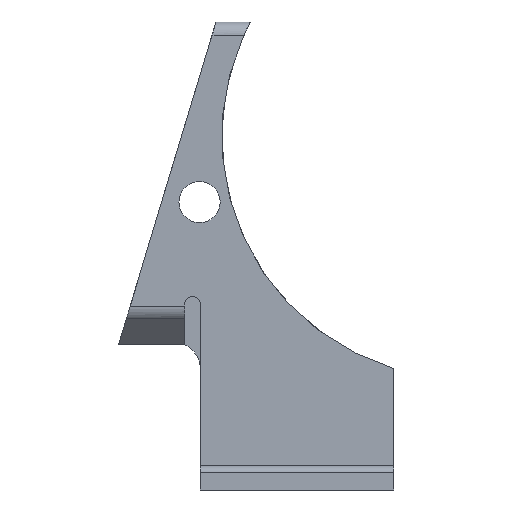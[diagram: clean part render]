
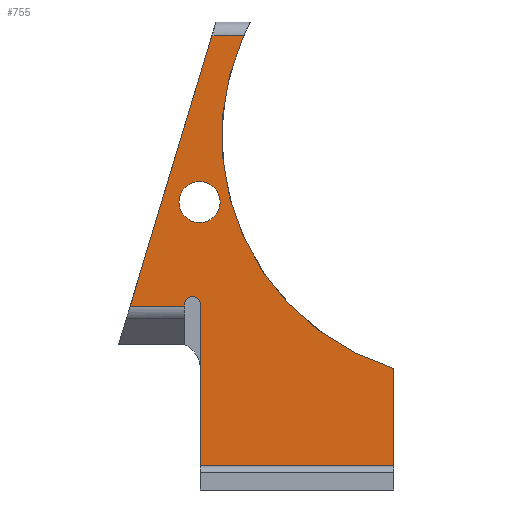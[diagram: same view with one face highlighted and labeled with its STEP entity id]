
A CAD part, left-side view. The second image highlights one B-rep face of the part: STEP entity #755.
In plain terms, the highlighted planar face has unit normal (-1, 0, 0).
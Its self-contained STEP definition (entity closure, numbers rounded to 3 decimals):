
#19=FACE_BOUND('',#89,.T.);
#24=PLANE('',#816);
#48=FACE_OUTER_BOUND('',#88,.T.);
#88=EDGE_LOOP('',(#528,#529,#530,#531,#532,#533,#534,#535,#536,#537,#538));
#89=EDGE_LOOP('',(#539));
#131=CIRCLE('',#817,0.5);
#132=CIRCLE('',#818,0.5);
#133=CIRCLE('',#819,17.951);
#134=CIRCLE('',#820,1.525);
#157=LINE('',#1112,#235);
#158=LINE('',#1115,#236);
#168=LINE('',#1145,#246);
#169=LINE('',#1149,#247);
#170=LINE('',#1153,#248);
#171=LINE('',#1155,#249);
#172=LINE('',#1157,#250);
#173=LINE('',#1160,#251);
#235=VECTOR('',#888,10.);
#236=VECTOR('',#891,10.);
#246=VECTOR('',#913,10.);
#247=VECTOR('',#916,10.);
#248=VECTOR('',#919,10.);
#249=VECTOR('',#920,10.);
#250=VECTOR('',#921,10.);
#251=VECTOR('',#924,10.);
#318=VERTEX_POINT('',#1105);
#321=VERTEX_POINT('',#1110);
#322=VERTEX_POINT('',#1114);
#336=VERTEX_POINT('',#1144);
#337=VERTEX_POINT('',#1146);
#338=VERTEX_POINT('',#1148);
#339=VERTEX_POINT('',#1150);
#340=VERTEX_POINT('',#1152);
#341=VERTEX_POINT('',#1154);
#342=VERTEX_POINT('',#1156);
#343=VERTEX_POINT('',#1158);
#344=VERTEX_POINT('',#1161);
#397=EDGE_CURVE('',#321,#318,#157,.T.);
#398=EDGE_CURVE('',#322,#318,#158,.T.);
#413=EDGE_CURVE('',#321,#336,#168,.T.);
#414=EDGE_CURVE('',#336,#337,#131,.T.);
#415=EDGE_CURVE('',#337,#338,#169,.T.);
#416=EDGE_CURVE('',#338,#339,#132,.T.);
#417=EDGE_CURVE('',#339,#340,#170,.T.);
#418=EDGE_CURVE('',#341,#340,#171,.T.);
#419=EDGE_CURVE('',#342,#341,#172,.T.);
#420=EDGE_CURVE('',#342,#343,#133,.T.);
#421=EDGE_CURVE('',#322,#343,#173,.T.);
#422=EDGE_CURVE('',#344,#344,#134,.T.);
#528=ORIENTED_EDGE('',*,*,#397,.F.);
#529=ORIENTED_EDGE('',*,*,#413,.T.);
#530=ORIENTED_EDGE('',*,*,#414,.T.);
#531=ORIENTED_EDGE('',*,*,#415,.T.);
#532=ORIENTED_EDGE('',*,*,#416,.T.);
#533=ORIENTED_EDGE('',*,*,#417,.T.);
#534=ORIENTED_EDGE('',*,*,#418,.F.);
#535=ORIENTED_EDGE('',*,*,#419,.F.);
#536=ORIENTED_EDGE('',*,*,#420,.T.);
#537=ORIENTED_EDGE('',*,*,#421,.F.);
#538=ORIENTED_EDGE('',*,*,#398,.T.);
#539=ORIENTED_EDGE('',*,*,#422,.T.);
#755=ADVANCED_FACE('',(#48,#19),#24,.T.);
#816=AXIS2_PLACEMENT_3D('',#1143,#911,#912);
#817=AXIS2_PLACEMENT_3D('',#1147,#914,#915);
#818=AXIS2_PLACEMENT_3D('',#1151,#917,#918);
#819=AXIS2_PLACEMENT_3D('',#1159,#922,#923);
#820=AXIS2_PLACEMENT_3D('',#1162,#925,#926);
#888=DIRECTION('',(0.,1.,0.));
#891=DIRECTION('',(0.,0.289,-0.957));
#911=DIRECTION('center_axis',(-1.,0.,0.));
#912=DIRECTION('ref_axis',(0.,0.,1.));
#913=DIRECTION('',(0.,0.,1.));
#914=DIRECTION('center_axis',(1.,0.,0.));
#915=DIRECTION('ref_axis',(0.,-1.,0.));
#916=DIRECTION('',(0.,-1.,0.));
#917=DIRECTION('center_axis',(1.,0.,0.));
#918=DIRECTION('ref_axis',(0.,-1.,0.));
#919=DIRECTION('',(0.,0.,-1.));
#920=DIRECTION('',(0.,1.,0.));
#921=DIRECTION('',(0.,0.,-1.));
#922=DIRECTION('center_axis',(1.,0.,0.));
#923=DIRECTION('ref_axis',(0.,-1.,0.));
#924=DIRECTION('',(0.,-1.,0.));
#925=DIRECTION('center_axis',(1.,0.,0.));
#926=DIRECTION('ref_axis',(0.,1.,0.));
#1105=CARTESIAN_POINT('',(-6.925,19.494,-19.731));
#1110=CARTESIAN_POINT('',(-6.925,15.45,-19.731));
#1112=CARTESIAN_POINT('',(-6.925,7.725,-19.731));
#1114=CARTESIAN_POINT('',(-6.925,13.442,0.3));
#1115=CARTESIAN_POINT('',(-6.925,17.207,-12.161));
#1143=CARTESIAN_POINT('Origin',(-6.925,0.,-32.05));
#1144=CARTESIAN_POINT('',(-6.925,15.45,-19.54));
#1145=CARTESIAN_POINT('',(-6.925,15.45,-26.045));
#1146=CARTESIAN_POINT('',(-6.925,14.95,-19.04));
#1147=CARTESIAN_POINT('Origin',(-6.925,14.95,-19.54));
#1148=CARTESIAN_POINT('',(-6.925,14.8,-19.04));
#1149=CARTESIAN_POINT('',(-6.925,7.475,-19.04));
#1150=CARTESIAN_POINT('',(-6.925,14.3,-19.54));
#1151=CARTESIAN_POINT('Origin',(-6.925,14.8,-19.54));
#1152=CARTESIAN_POINT('',(-6.925,14.3,-31.55));
#1153=CARTESIAN_POINT('',(-6.925,14.3,-27.225));
#1154=CARTESIAN_POINT('',(-6.925,0.,-31.55));
#1155=CARTESIAN_POINT('',(-6.925,0.,-31.55));
#1156=CARTESIAN_POINT('',(-6.925,0.,-24.35));
#1157=CARTESIAN_POINT('',(-6.925,0.,1.3));
#1158=CARTESIAN_POINT('',(-6.925,11.086,0.3));
#1159=CARTESIAN_POINT('Origin',(-6.925,-5.234,-7.178));
#1160=CARTESIAN_POINT('',(-6.925,0.,0.3));
#1161=CARTESIAN_POINT('',(-6.925,12.833,-12.038));
#1162=CARTESIAN_POINT('Origin',(-6.925,14.358,-12.038));
